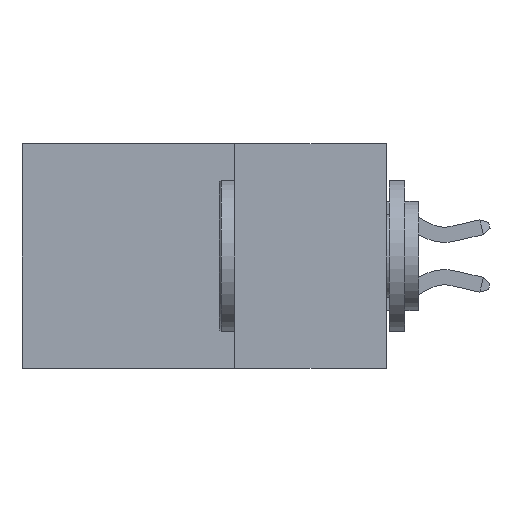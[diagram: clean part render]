
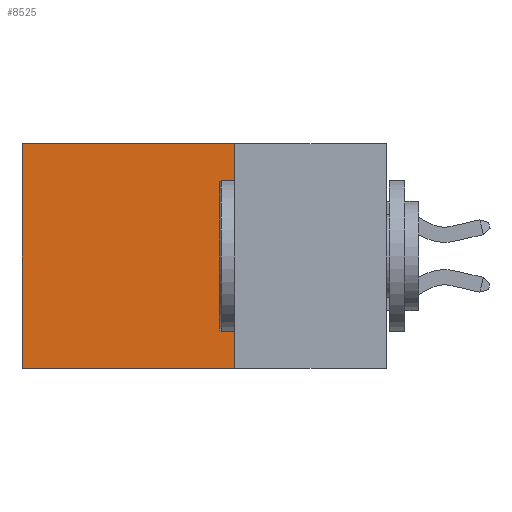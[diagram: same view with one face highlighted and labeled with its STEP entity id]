
A CAD part, left-side view. The second image highlights one B-rep face of the part: STEP entity #8525.
In plain terms, the highlighted planar face has unit normal (-1, 0, 0).
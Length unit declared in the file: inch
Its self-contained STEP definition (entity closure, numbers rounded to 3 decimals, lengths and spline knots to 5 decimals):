
#14 = CARTESIAN_POINT ( 'NONE',  ( 0.2615, 0.25, -0.37 ) ) ;
#705 = DIRECTION ( 'NONE',  ( 0., 0., -1. ) ) ;
#1428 = CARTESIAN_POINT ( 'NONE',  ( 0.2615, 0.25, -0.37 ) ) ;
#1545 = PLANE ( 'NONE',  #7735 ) ;
#2826 = CARTESIAN_POINT ( 'NONE',  ( 0.2615, 0.6, -0.37 ) ) ;
#5008 = CARTESIAN_POINT ( 'NONE',  ( 0.2615, 0.25, 0. ) ) ;
#5349 = DIRECTION ( 'NONE',  ( 0., 0., -1. ) ) ;
#6034 = LINE ( 'NONE', #2826, #14864 ) ;
#6316 = DIRECTION ( 'NONE',  ( 0., 1., 0. ) ) ;
#6369 = ORIENTED_EDGE ( 'NONE', *, *, #18309, .T. ) ;
#7111 = DIRECTION ( 'NONE',  ( 0., 0., -1. ) ) ;
#7478 = ORIENTED_EDGE ( 'NONE', *, *, #8971, .T. ) ;
#7735 = AXIS2_PLACEMENT_3D ( 'NONE', #1428, #21131, #7111 ) ;
#8037 = EDGE_LOOP ( 'NONE', ( #7478, #12815, #17428, #6369 ) ) ;
#8525 = ADVANCED_FACE ( 'NONE', ( #14296 ), #1545, .F. ) ;
#8971 = EDGE_CURVE ( 'NONE', #17140, #12865, #6034, .T. ) ;
#12467 = LINE ( 'NONE', #14899, #21801 ) ;
#12815 = ORIENTED_EDGE ( 'NONE', *, *, #14151, .F. ) ;
#12865 = VERTEX_POINT ( 'NONE', #13665 ) ;
#13565 = CARTESIAN_POINT ( 'NONE',  ( 0.2615, 0.25, 0. ) ) ;
#13580 = VECTOR ( 'NONE', #5349, 39.37008 ) ;
#13665 = CARTESIAN_POINT ( 'NONE',  ( 0.2615, 0.6, -0.37 ) ) ;
#13671 = DIRECTION ( 'NONE',  ( 0., 1., 0. ) ) ;
#14151 = EDGE_CURVE ( 'NONE', #19935, #12865, #12467, .T. ) ;
#14296 = FACE_OUTER_BOUND ( 'NONE', #8037, .T. ) ;
#14307 = LINE ( 'NONE', #14, #13580 ) ;
#14864 = VECTOR ( 'NONE', #705, 39.37008 ) ;
#14899 = CARTESIAN_POINT ( 'NONE',  ( 0.2615, 0.25, -0.37 ) ) ;
#15695 = CARTESIAN_POINT ( 'NONE',  ( 0.2615, 0.25, -0.37 ) ) ;
#17140 = VERTEX_POINT ( 'NONE', #21631 ) ;
#17428 = ORIENTED_EDGE ( 'NONE', *, *, #22233, .F. ) ;
#18008 = VERTEX_POINT ( 'NONE', #5008 ) ;
#18309 = EDGE_CURVE ( 'NONE', #18008, #17140, #21192, .T. ) ;
#19534 = VECTOR ( 'NONE', #13671, 39.37008 ) ;
#19935 = VERTEX_POINT ( 'NONE', #15695 ) ;
#21131 = DIRECTION ( 'NONE',  ( 1., 0., 0. ) ) ;
#21192 = LINE ( 'NONE', #13565, #19534 ) ;
#21631 = CARTESIAN_POINT ( 'NONE',  ( 0.2615, 0.6, 0. ) ) ;
#21801 = VECTOR ( 'NONE', #6316, 39.37008 ) ;
#22233 = EDGE_CURVE ( 'NONE', #18008, #19935, #14307, .T. ) ;
